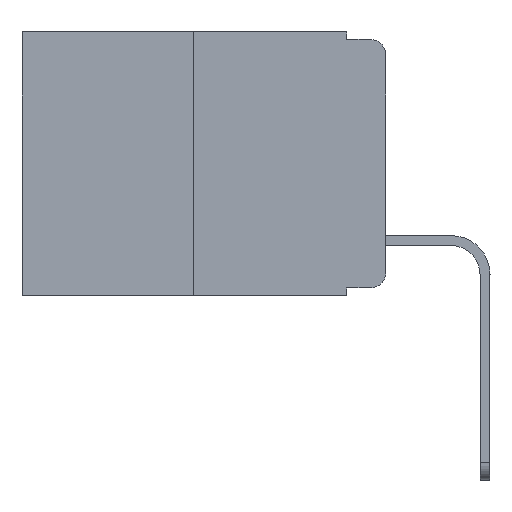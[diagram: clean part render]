
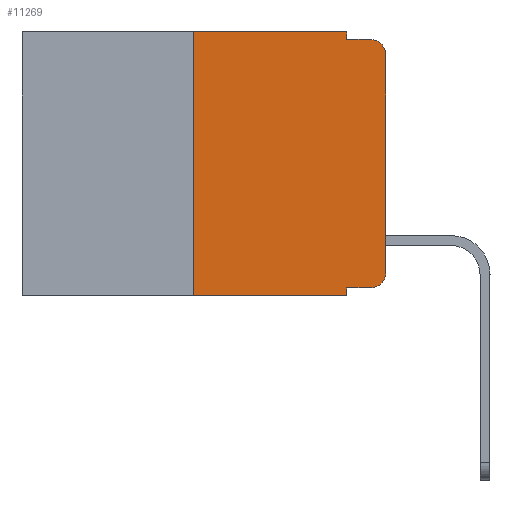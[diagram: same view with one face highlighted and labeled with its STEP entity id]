
A CAD part, left-side view. The second image highlights one B-rep face of the part: STEP entity #11269.
In plain terms, the highlighted planar face has unit normal (-1, 0, 0).
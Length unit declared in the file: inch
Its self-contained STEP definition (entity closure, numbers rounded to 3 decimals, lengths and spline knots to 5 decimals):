
#102 = CARTESIAN_POINT ( 'NONE',  ( 0., 0.25, 0. ) ) ;
#372 = ORIENTED_EDGE ( 'NONE', *, *, #20329, .F. ) ;
#479 = DIRECTION ( 'NONE',  ( 0., -1., 0. ) ) ;
#504 = LINE ( 'NONE', #102, #3809 ) ;
#506 = DIRECTION ( 'NONE',  ( -1., 0., 0. ) ) ;
#661 = ORIENTED_EDGE ( 'NONE', *, *, #2283, .T. ) ;
#836 = DIRECTION ( 'NONE',  ( 0., 0., -1. ) ) ;
#907 = ORIENTED_EDGE ( 'NONE', *, *, #8386, .F. ) ;
#1032 = CARTESIAN_POINT ( 'NONE',  ( 0., 0.051, 0. ) ) ;
#1137 = VERTEX_POINT ( 'NONE', #7171 ) ;
#1190 = DIRECTION ( 'NONE',  ( 1., 0., 0. ) ) ;
#1370 = FACE_OUTER_BOUND ( 'NONE', #10583, .T. ) ;
#1714 = VERTEX_POINT ( 'NONE', #19292 ) ;
#1877 = EDGE_CURVE ( 'NONE', #7846, #19308, #3395, .T. ) ;
#1947 = CARTESIAN_POINT ( 'NONE',  ( 0., 0.02, -0.313 ) ) ;
#2025 = EDGE_CURVE ( 'NONE', #12311, #4345, #12355, .T. ) ;
#2283 = EDGE_CURVE ( 'NONE', #18630, #19308, #7216, .T. ) ;
#2298 = CARTESIAN_POINT ( 'NONE',  ( 0., 0.051, -0.333 ) ) ;
#2311 = EDGE_CURVE ( 'NONE', #7846, #13429, #20754, .T. ) ;
#2615 = LINE ( 'NONE', #7013, #5935 ) ;
#2816 = CARTESIAN_POINT ( 'NONE',  ( 0., 0.051, 0. ) ) ;
#3395 = LINE ( 'NONE', #2816, #15912 ) ;
#3558 = EDGE_CURVE ( 'NONE', #13429, #1137, #17113, .T. ) ;
#3809 = VECTOR ( 'NONE', #9629, 39.37008 ) ;
#4114 = VECTOR ( 'NONE', #12194, 39.37008 ) ;
#4147 = CARTESIAN_POINT ( 'NONE',  ( 0., 0.051, -0.343 ) ) ;
#4345 = VERTEX_POINT ( 'NONE', #10506 ) ;
#5225 = DIRECTION ( 'NONE',  ( 0., 0., -1. ) ) ;
#5935 = VECTOR ( 'NONE', #11454, 39.37008 ) ;
#6746 = LINE ( 'NONE', #16495, #19791 ) ;
#6767 = LINE ( 'NONE', #1032, #9083 ) ;
#7013 = CARTESIAN_POINT ( 'NONE',  ( 0., 0.473, 0. ) ) ;
#7171 = CARTESIAN_POINT ( 'NONE',  ( 0., 0., -0.313 ) ) ;
#7198 = CARTESIAN_POINT ( 'NONE',  ( 0., 0.25, -0.343 ) ) ;
#7216 = LINE ( 'NONE', #10562, #4114 ) ;
#7846 = VERTEX_POINT ( 'NONE', #2298 ) ;
#7863 = ORIENTED_EDGE ( 'NONE', *, *, #19707, .T. ) ;
#8386 = EDGE_CURVE ( 'NONE', #18630, #20211, #504, .T. ) ;
#9001 = CARTESIAN_POINT ( 'NONE',  ( 0., 0.02, -0.03 ) ) ;
#9083 = VECTOR ( 'NONE', #836, 39.37008 ) ;
#9629 = DIRECTION ( 'NONE',  ( 0., 0., 1. ) ) ;
#9865 = CIRCLE ( 'NONE', #14027, 0.02 ) ;
#10082 = ORIENTED_EDGE ( 'NONE', *, *, #2025, .F. ) ;
#10435 = CARTESIAN_POINT ( 'NONE',  ( 0., 0.051, -0.333 ) ) ;
#10506 = CARTESIAN_POINT ( 'NONE',  ( 0., 0.02, -0.01 ) ) ;
#10562 = CARTESIAN_POINT ( 'NONE',  ( 0., 0.473, -0.343 ) ) ;
#10583 = EDGE_LOOP ( 'NONE', ( #7863, #15237, #10082, #16477, #372, #907, #661, #12887, #18237, #16110 ) ) ;
#10614 = EDGE_CURVE ( 'NONE', #19397, #4345, #9865, .T. ) ;
#10980 = CARTESIAN_POINT ( 'NONE',  ( 0., 0.473, 0. ) ) ;
#11269 = ADVANCED_FACE ( 'NONE', ( #1370 ), #19103, .F. ) ;
#11340 = VECTOR ( 'NONE', #13046, 39.37008 ) ;
#11425 = CARTESIAN_POINT ( 'NONE',  ( 0., 0.051, -0.01 ) ) ;
#11454 = DIRECTION ( 'NONE',  ( 0., -1., 0. ) ) ;
#11688 = DIRECTION ( 'NONE',  ( 0., 0., 1. ) ) ;
#11945 = DIRECTION ( 'NONE',  ( 0., 0., -1. ) ) ;
#12161 = AXIS2_PLACEMENT_3D ( 'NONE', #1947, #18205, #5225 ) ;
#12194 = DIRECTION ( 'NONE',  ( 0., -1., 0. ) ) ;
#12311 = VERTEX_POINT ( 'NONE', #20001 ) ;
#12355 = LINE ( 'NONE', #11425, #11340 ) ;
#12612 = DIRECTION ( 'NONE',  ( 0., 0., -1. ) ) ;
#12887 = ORIENTED_EDGE ( 'NONE', *, *, #1877, .F. ) ;
#13046 = DIRECTION ( 'NONE',  ( 0., -1., 0. ) ) ;
#13429 = VERTEX_POINT ( 'NONE', #14299 ) ;
#14027 = AXIS2_PLACEMENT_3D ( 'NONE', #9001, #506, #11945 ) ;
#14299 = CARTESIAN_POINT ( 'NONE',  ( 0., 0.02, -0.333 ) ) ;
#14787 = CARTESIAN_POINT ( 'NONE',  ( 0., 0.25, 0. ) ) ;
#15237 = ORIENTED_EDGE ( 'NONE', *, *, #10614, .T. ) ;
#15912 = VECTOR ( 'NONE', #19341, 39.37008 ) ;
#16110 = ORIENTED_EDGE ( 'NONE', *, *, #3558, .T. ) ;
#16477 = ORIENTED_EDGE ( 'NONE', *, *, #19335, .F. ) ;
#16495 = CARTESIAN_POINT ( 'NONE',  ( 0., 0., 0. ) ) ;
#17113 = CIRCLE ( 'NONE', #12161, 0.02 ) ;
#17861 = AXIS2_PLACEMENT_3D ( 'NONE', #10980, #1190, #12612 ) ;
#18205 = DIRECTION ( 'NONE',  ( -1., 0., 0. ) ) ;
#18237 = ORIENTED_EDGE ( 'NONE', *, *, #2311, .T. ) ;
#18630 = VERTEX_POINT ( 'NONE', #7198 ) ;
#19103 = PLANE ( 'NONE',  #17861 ) ;
#19229 = VECTOR ( 'NONE', #479, 39.37008 ) ;
#19292 = CARTESIAN_POINT ( 'NONE',  ( 0., 0.051, 0. ) ) ;
#19308 = VERTEX_POINT ( 'NONE', #4147 ) ;
#19323 = CARTESIAN_POINT ( 'NONE',  ( 0., 0., -0.03 ) ) ;
#19335 = EDGE_CURVE ( 'NONE', #1714, #12311, #6767, .T. ) ;
#19341 = DIRECTION ( 'NONE',  ( 0., 0., -1. ) ) ;
#19397 = VERTEX_POINT ( 'NONE', #19323 ) ;
#19707 = EDGE_CURVE ( 'NONE', #1137, #19397, #6746, .T. ) ;
#19791 = VECTOR ( 'NONE', #11688, 39.37008 ) ;
#20001 = CARTESIAN_POINT ( 'NONE',  ( 0., 0.051, -0.01 ) ) ;
#20211 = VERTEX_POINT ( 'NONE', #14787 ) ;
#20329 = EDGE_CURVE ( 'NONE', #20211, #1714, #2615, .T. ) ;
#20754 = LINE ( 'NONE', #10435, #19229 ) ;
